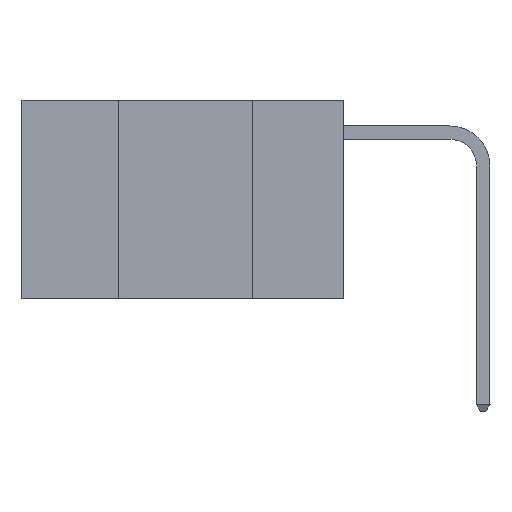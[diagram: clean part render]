
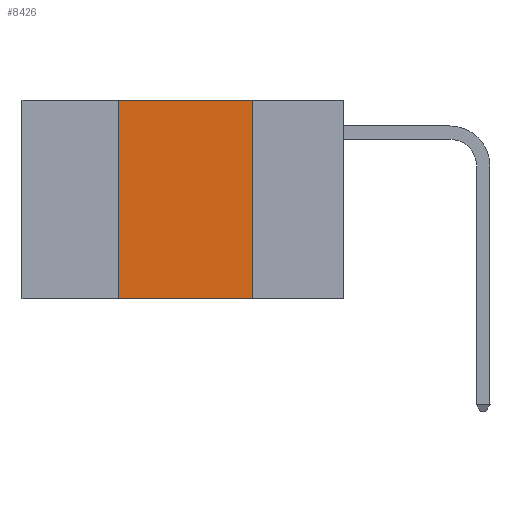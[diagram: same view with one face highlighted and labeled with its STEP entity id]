
A CAD part, left-side view. The second image highlights one B-rep face of the part: STEP entity #8426.
In plain terms, the highlighted planar face has unit normal (-1, 0, 0).
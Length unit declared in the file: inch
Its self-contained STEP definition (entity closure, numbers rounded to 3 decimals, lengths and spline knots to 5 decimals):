
#83 = ORIENTED_EDGE ( 'NONE', *, *, #5730, .F. ) ;
#140 = CARTESIAN_POINT ( 'NONE',  ( 0., 0.6, 0. ) ) ;
#524 = ORIENTED_EDGE ( 'NONE', *, *, #1993, .F. ) ;
#622 = CARTESIAN_POINT ( 'NONE',  ( 0., 0.17, 0. ) ) ;
#652 = ORIENTED_EDGE ( 'NONE', *, *, #7818, .F. ) ;
#896 = ORIENTED_EDGE ( 'NONE', *, *, #9169, .T. ) ;
#995 = DIRECTION ( 'NONE',  ( 0., 0., -1. ) ) ;
#1096 = FACE_OUTER_BOUND ( 'NONE', #3445, .T. ) ;
#1212 = VERTEX_POINT ( 'NONE', #622 ) ;
#1280 = VERTEX_POINT ( 'NONE', #9741 ) ;
#1785 = LINE ( 'NONE', #9590, #2583 ) ;
#1993 = EDGE_CURVE ( 'NONE', #2043, #1212, #5977, .T. ) ;
#2043 = VERTEX_POINT ( 'NONE', #8510 ) ;
#2583 = VECTOR ( 'NONE', #6733, 39.37008 ) ;
#2792 = CARTESIAN_POINT ( 'NONE',  ( 0., 0.17, 0. ) ) ;
#3445 = EDGE_LOOP ( 'NONE', ( #83, #524, #652, #896 ) ) ;
#4419 = DIRECTION ( 'NONE',  ( 0., 0., 1. ) ) ;
#5284 = CARTESIAN_POINT ( 'NONE',  ( 0., 0.42, -0.37 ) ) ;
#5730 = EDGE_CURVE ( 'NONE', #1212, #1280, #7769, .T. ) ;
#5828 = DIRECTION ( 'NONE',  ( 1., 0., 0. ) ) ;
#5977 = LINE ( 'NONE', #8882, #6089 ) ;
#6089 = VECTOR ( 'NONE', #8911, 39.37008 ) ;
#6460 = VERTEX_POINT ( 'NONE', #5284 ) ;
#6733 = DIRECTION ( 'NONE',  ( 0., -1., 0. ) ) ;
#7187 = LINE ( 'NONE', #9576, #8503 ) ;
#7432 = DIRECTION ( 'NONE',  ( 0., 0., -1. ) ) ;
#7546 = AXIS2_PLACEMENT_3D ( 'NONE', #140, #5828, #995 ) ;
#7769 = LINE ( 'NONE', #2792, #9607 ) ;
#7818 = EDGE_CURVE ( 'NONE', #6460, #2043, #7187, .T. ) ;
#8426 = ADVANCED_FACE ( 'NONE', ( #1096 ), #8754, .F. ) ;
#8503 = VECTOR ( 'NONE', #4419, 39.37008 ) ;
#8510 = CARTESIAN_POINT ( 'NONE',  ( 0., 0.42, 0. ) ) ;
#8754 = PLANE ( 'NONE',  #7546 ) ;
#8882 = CARTESIAN_POINT ( 'NONE',  ( 0., 0.6, 0. ) ) ;
#8911 = DIRECTION ( 'NONE',  ( 0., -1., 0. ) ) ;
#9169 = EDGE_CURVE ( 'NONE', #6460, #1280, #1785, .T. ) ;
#9576 = CARTESIAN_POINT ( 'NONE',  ( 0., 0.42, 0. ) ) ;
#9590 = CARTESIAN_POINT ( 'NONE',  ( 0., 0.6, -0.37 ) ) ;
#9607 = VECTOR ( 'NONE', #7432, 39.37008 ) ;
#9741 = CARTESIAN_POINT ( 'NONE',  ( 0., 0.17, -0.37 ) ) ;
